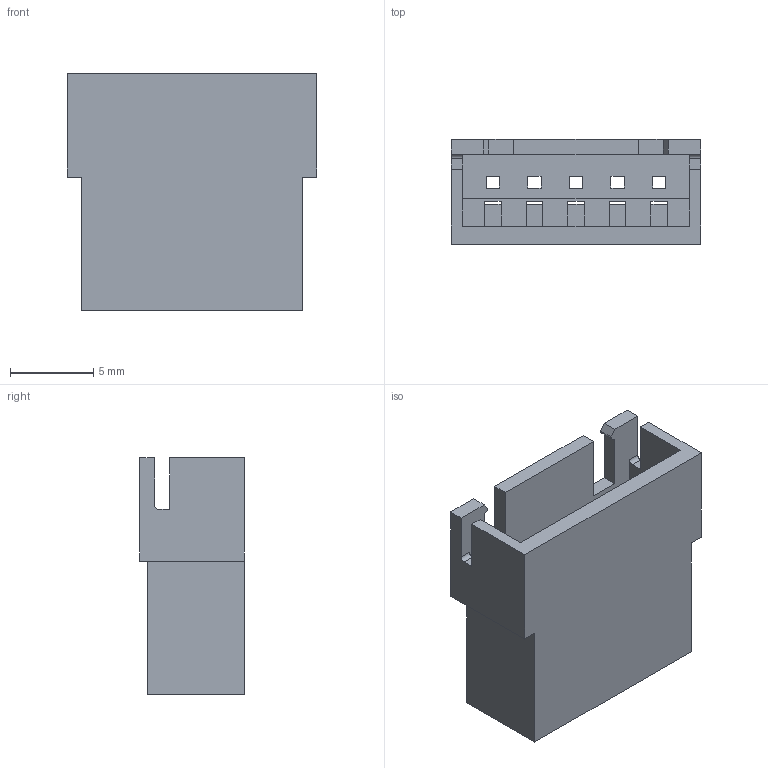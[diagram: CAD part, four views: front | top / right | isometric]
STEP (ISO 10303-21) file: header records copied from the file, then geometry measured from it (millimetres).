
FILE_DESCRIPTION (( 'STEP AP203' ), '1' );
FILE_NAME ('14K-505-210-AA1.STEP', '2024-02-23T14:31:32', ( '' ), ( '' ), 'SwSTEP 2.0', 'SolidWorks 2023', '' );
FILE_SCHEMA (( 'CONFIG_CONTROL_DESIGN' ));
Length unit declared in the file: millimetre
Products named in the file (1): 14K-505-210-AA1
Bounding box: 15 x 6.3 x 14.2 mm (x, y, z)
Volume: 636.1 mm3; surface area: 1472.3 mm2
Topology: 1 solids, 1 shells, 164 faces, 488 edges, 322 vertices
Faces by surface type: plane 160, cylinder 4
Entity records: 5497 total; most frequent: ORIENTED_EDGE 976, CARTESIAN_POINT 975, DIRECTION 826, EDGE_CURVE 488, VECTOR 480, LINE 480, VERTEX_POINT 322, EDGE_LOOP 180
